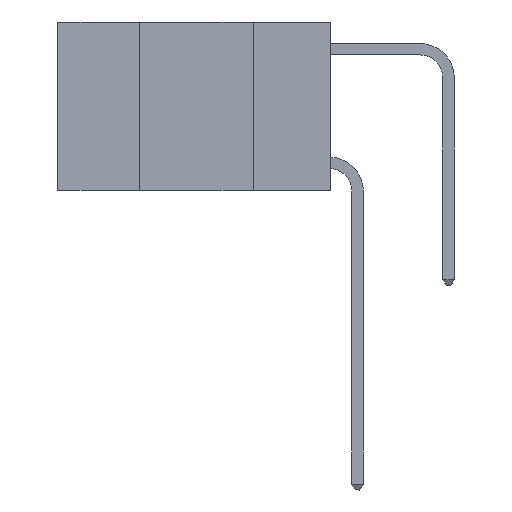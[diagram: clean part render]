
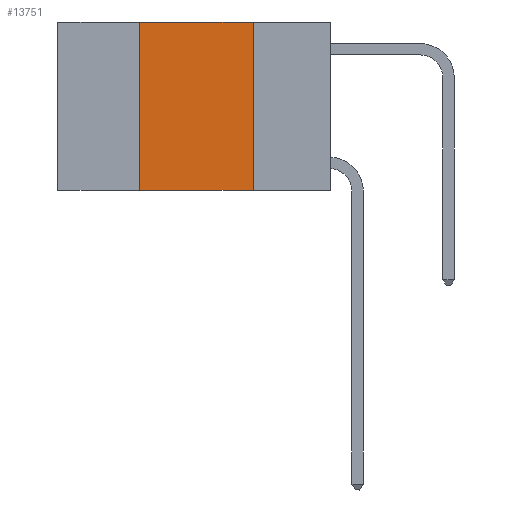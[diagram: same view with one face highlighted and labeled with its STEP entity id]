
A CAD part, left-side view. The second image highlights one B-rep face of the part: STEP entity #13751.
In plain terms, the highlighted planar face has unit normal (-1, 0, 0).
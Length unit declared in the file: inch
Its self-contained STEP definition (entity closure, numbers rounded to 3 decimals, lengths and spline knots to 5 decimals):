
#2 = LINE ( 'NONE', #12072, #6740 ) ;
#594 = LINE ( 'NONE', #10803, #3534 ) ;
#724 = DIRECTION ( 'NONE',  ( 0., -1., 0. ) ) ;
#891 = FACE_OUTER_BOUND ( 'NONE', #4712, .T. ) ;
#1401 = ORIENTED_EDGE ( 'NONE', *, *, #9443, .F. ) ;
#1964 = VECTOR ( 'NONE', #4604, 39.37008 ) ;
#2573 = LINE ( 'NONE', #4405, #5960 ) ;
#3048 = CARTESIAN_POINT ( 'NONE',  ( 0., 0.6, 0. ) ) ;
#3534 = VECTOR ( 'NONE', #4336, 39.37008 ) ;
#4317 = DIRECTION ( 'NONE',  ( 0., 0., -1. ) ) ;
#4336 = DIRECTION ( 'NONE',  ( 0., 0., 1. ) ) ;
#4405 = CARTESIAN_POINT ( 'NONE',  ( 0., 0.6, 0. ) ) ;
#4427 = DIRECTION ( 'NONE',  ( 0., 0., -1. ) ) ;
#4604 = DIRECTION ( 'NONE',  ( 0., -1., 0. ) ) ;
#4712 = EDGE_LOOP ( 'NONE', ( #5949, #1401, #12516, #8347 ) ) ;
#5308 = LINE ( 'NONE', #13449, #1964 ) ;
#5948 = VERTEX_POINT ( 'NONE', #13022 ) ;
#5949 = ORIENTED_EDGE ( 'NONE', *, *, #15604, .F. ) ;
#5960 = VECTOR ( 'NONE', #724, 39.37008 ) ;
#6740 = VECTOR ( 'NONE', #4427, 39.37008 ) ;
#7855 = VERTEX_POINT ( 'NONE', #15513 ) ;
#8347 = ORIENTED_EDGE ( 'NONE', *, *, #10599, .T. ) ;
#9443 = EDGE_CURVE ( 'NONE', #15209, #5948, #2573, .T. ) ;
#9924 = CARTESIAN_POINT ( 'NONE',  ( 0., 0.42, 0. ) ) ;
#10038 = CARTESIAN_POINT ( 'NONE',  ( 0., 0.17, -0.37 ) ) ;
#10499 = EDGE_CURVE ( 'NONE', #7855, #15209, #594, .T. ) ;
#10599 = EDGE_CURVE ( 'NONE', #7855, #10812, #5308, .T. ) ;
#10803 = CARTESIAN_POINT ( 'NONE',  ( 0., 0.42, 0. ) ) ;
#10812 = VERTEX_POINT ( 'NONE', #10038 ) ;
#11965 = DIRECTION ( 'NONE',  ( 1., 0., 0. ) ) ;
#12072 = CARTESIAN_POINT ( 'NONE',  ( 0., 0.17, 0. ) ) ;
#12516 = ORIENTED_EDGE ( 'NONE', *, *, #10499, .F. ) ;
#13022 = CARTESIAN_POINT ( 'NONE',  ( 0., 0.17, 0. ) ) ;
#13152 = PLANE ( 'NONE',  #13997 ) ;
#13449 = CARTESIAN_POINT ( 'NONE',  ( 0., 0.6, -0.37 ) ) ;
#13751 = ADVANCED_FACE ( 'NONE', ( #891 ), #13152, .F. ) ;
#13997 = AXIS2_PLACEMENT_3D ( 'NONE', #3048, #11965, #4317 ) ;
#15209 = VERTEX_POINT ( 'NONE', #9924 ) ;
#15513 = CARTESIAN_POINT ( 'NONE',  ( 0., 0.42, -0.37 ) ) ;
#15604 = EDGE_CURVE ( 'NONE', #5948, #10812, #2, .T. ) ;
